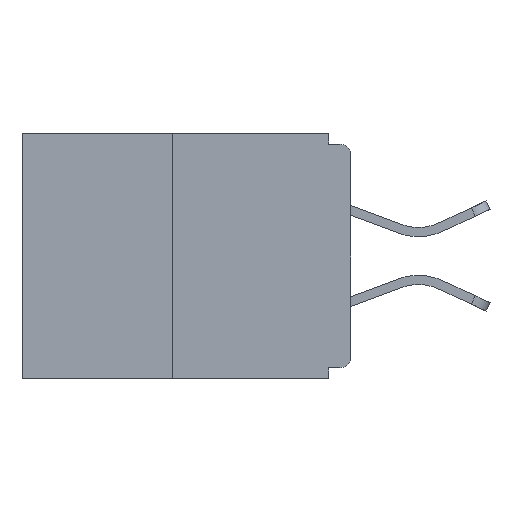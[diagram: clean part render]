
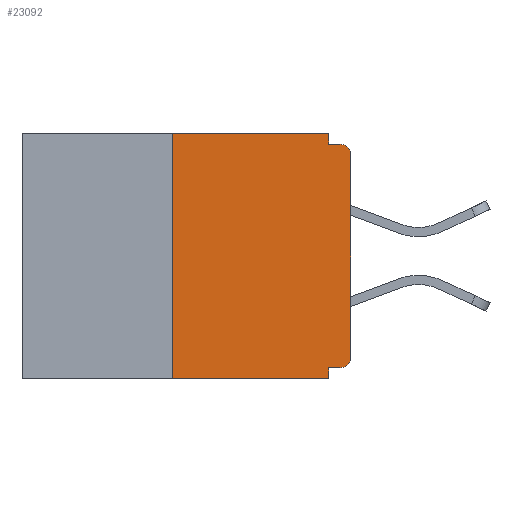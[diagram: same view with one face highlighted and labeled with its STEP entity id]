
A CAD part, left-side view. The second image highlights one B-rep face of the part: STEP entity #23092.
In plain terms, the highlighted planar face has unit normal (-1, 0, 0).
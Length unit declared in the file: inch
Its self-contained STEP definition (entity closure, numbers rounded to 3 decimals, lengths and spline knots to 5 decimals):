
#216 = AXIS2_PLACEMENT_3D ( 'NONE', #4070, #10775, #8412 ) ;
#512 = ORIENTED_EDGE ( 'NONE', *, *, #7040, .T. ) ;
#782 = VERTEX_POINT ( 'NONE', #23064 ) ;
#1122 = CARTESIAN_POINT ( 'NONE',  ( 0., 0., -0.313 ) ) ;
#1650 = LINE ( 'NONE', #24889, #19597 ) ;
#1940 = ORIENTED_EDGE ( 'NONE', *, *, #14724, .T. ) ;
#2134 = CARTESIAN_POINT ( 'NONE',  ( 0., 0.031, 0. ) ) ;
#2149 = CARTESIAN_POINT ( 'NONE',  ( 0., 0.031, 0. ) ) ;
#2177 = CARTESIAN_POINT ( 'NONE',  ( 0., 0.015, -0.328 ) ) ;
#2659 = CARTESIAN_POINT ( 'NONE',  ( 0., 0.031, -0.343 ) ) ;
#2739 = ORIENTED_EDGE ( 'NONE', *, *, #7778, .F. ) ;
#3153 = CARTESIAN_POINT ( 'NONE',  ( 0., 0., 0. ) ) ;
#3610 = EDGE_LOOP ( 'NONE', ( #26290, #14621, #512, #16430, #17605, #1940, #14262, #9867, #25246, #2739 ) ) ;
#4059 = VECTOR ( 'NONE', #20643, 39.37008 ) ;
#4070 = CARTESIAN_POINT ( 'NONE',  ( 0., 0.015, -0.03 ) ) ;
#4645 = LINE ( 'NONE', #3153, #14335 ) ;
#4896 = CARTESIAN_POINT ( 'NONE',  ( 0., 0.25, -0.343 ) ) ;
#6664 = CARTESIAN_POINT ( 'NONE',  ( 0., 0.031, -0.015 ) ) ;
#6713 = VECTOR ( 'NONE', #24167, 39.37008 ) ;
#6939 = VECTOR ( 'NONE', #21904, 39.37008 ) ;
#7040 = EDGE_CURVE ( 'NONE', #17635, #20829, #14366, .T. ) ;
#7135 = DIRECTION ( 'NONE',  ( 0., -1., 0. ) ) ;
#7186 = CARTESIAN_POINT ( 'NONE',  ( 0., 0., -0.03 ) ) ;
#7405 = CARTESIAN_POINT ( 'NONE',  ( 0., 0.031, -0.343 ) ) ;
#7778 = EDGE_CURVE ( 'NONE', #22072, #26523, #17300, .T. ) ;
#8412 = DIRECTION ( 'NONE',  ( 0., 0., -1. ) ) ;
#9184 = VECTOR ( 'NONE', #24352, 39.37008 ) ;
#9346 = EDGE_CURVE ( 'NONE', #26523, #9687, #1650, .T. ) ;
#9687 = VERTEX_POINT ( 'NONE', #26126 ) ;
#9867 = ORIENTED_EDGE ( 'NONE', *, *, #16054, .T. ) ;
#10696 = CARTESIAN_POINT ( 'NONE',  ( 0., 0., -0.328 ) ) ;
#10775 = DIRECTION ( 'NONE',  ( -1., 0., 0. ) ) ;
#11550 = VERTEX_POINT ( 'NONE', #2177 ) ;
#12062 = CIRCLE ( 'NONE', #216, 0.015 ) ;
#12261 = FACE_OUTER_BOUND ( 'NONE', #3610, .T. ) ;
#12551 = CARTESIAN_POINT ( 'NONE',  ( 0., 0.46, -0.343 ) ) ;
#12884 = VERTEX_POINT ( 'NONE', #14069 ) ;
#13541 = AXIS2_PLACEMENT_3D ( 'NONE', #19665, #26237, #17625 ) ;
#14069 = CARTESIAN_POINT ( 'NONE',  ( 0., 0.25, 0. ) ) ;
#14262 = ORIENTED_EDGE ( 'NONE', *, *, #18339, .T. ) ;
#14335 = VECTOR ( 'NONE', #22857, 39.37008 ) ;
#14366 = LINE ( 'NONE', #12551, #19481 ) ;
#14621 = ORIENTED_EDGE ( 'NONE', *, *, #17819, .F. ) ;
#14724 = EDGE_CURVE ( 'NONE', #11550, #15999, #20383, .T. ) ;
#15032 = PLANE ( 'NONE',  #13541 ) ;
#15458 = LINE ( 'NONE', #10696, #23035 ) ;
#15999 = VERTEX_POINT ( 'NONE', #1122 ) ;
#16054 = EDGE_CURVE ( 'NONE', #16461, #9687, #12062, .T. ) ;
#16430 = ORIENTED_EDGE ( 'NONE', *, *, #17110, .F. ) ;
#16450 = LINE ( 'NONE', #2659, #9184 ) ;
#16461 = VERTEX_POINT ( 'NONE', #7186 ) ;
#16693 = DIRECTION ( 'NONE',  ( -1., 0., 0. ) ) ;
#17110 = EDGE_CURVE ( 'NONE', #782, #20829, #16450, .T. ) ;
#17227 = AXIS2_PLACEMENT_3D ( 'NONE', #21120, #16693, #20928 ) ;
#17300 = LINE ( 'NONE', #2134, #6939 ) ;
#17605 = ORIENTED_EDGE ( 'NONE', *, *, #20961, .F. ) ;
#17612 = CARTESIAN_POINT ( 'NONE',  ( 0., 0.25, 0. ) ) ;
#17625 = DIRECTION ( 'NONE',  ( 0., 0., -1. ) ) ;
#17635 = VERTEX_POINT ( 'NONE', #4896 ) ;
#17819 = EDGE_CURVE ( 'NONE', #17635, #12884, #26767, .T. ) ;
#18339 = EDGE_CURVE ( 'NONE', #15999, #16461, #4645, .T. ) ;
#18502 = CARTESIAN_POINT ( 'NONE',  ( 0., 0.46, 0. ) ) ;
#19481 = VECTOR ( 'NONE', #27989, 39.37008 ) ;
#19572 = LINE ( 'NONE', #18502, #4059 ) ;
#19597 = VECTOR ( 'NONE', #7135, 39.37008 ) ;
#19665 = CARTESIAN_POINT ( 'NONE',  ( 0., 0.46, 0. ) ) ;
#20383 = CIRCLE ( 'NONE', #17227, 0.015 ) ;
#20643 = DIRECTION ( 'NONE',  ( 0., -1., 0. ) ) ;
#20796 = EDGE_CURVE ( 'NONE', #12884, #22072, #19572, .T. ) ;
#20829 = VERTEX_POINT ( 'NONE', #7405 ) ;
#20928 = DIRECTION ( 'NONE',  ( 0., 0., -1. ) ) ;
#20961 = EDGE_CURVE ( 'NONE', #11550, #782, #15458, .T. ) ;
#21120 = CARTESIAN_POINT ( 'NONE',  ( 0., 0.015, -0.313 ) ) ;
#21904 = DIRECTION ( 'NONE',  ( 0., 0., -1. ) ) ;
#22072 = VERTEX_POINT ( 'NONE', #2149 ) ;
#22857 = DIRECTION ( 'NONE',  ( 0., 0., 1. ) ) ;
#23035 = VECTOR ( 'NONE', #23499, 39.37008 ) ;
#23064 = CARTESIAN_POINT ( 'NONE',  ( 0., 0.031, -0.328 ) ) ;
#23092 = ADVANCED_FACE ( 'NONE', ( #12261 ), #15032, .F. ) ;
#23499 = DIRECTION ( 'NONE',  ( 0., 1., 0. ) ) ;
#24167 = DIRECTION ( 'NONE',  ( 0., 0., 1. ) ) ;
#24352 = DIRECTION ( 'NONE',  ( 0., 0., -1. ) ) ;
#24889 = CARTESIAN_POINT ( 'NONE',  ( 0., 0., -0.015 ) ) ;
#25246 = ORIENTED_EDGE ( 'NONE', *, *, #9346, .F. ) ;
#26126 = CARTESIAN_POINT ( 'NONE',  ( 0., 0.015, -0.015 ) ) ;
#26237 = DIRECTION ( 'NONE',  ( 1., 0., 0. ) ) ;
#26290 = ORIENTED_EDGE ( 'NONE', *, *, #20796, .F. ) ;
#26523 = VERTEX_POINT ( 'NONE', #6664 ) ;
#26767 = LINE ( 'NONE', #17612, #6713 ) ;
#27989 = DIRECTION ( 'NONE',  ( 0., -1., 0. ) ) ;
